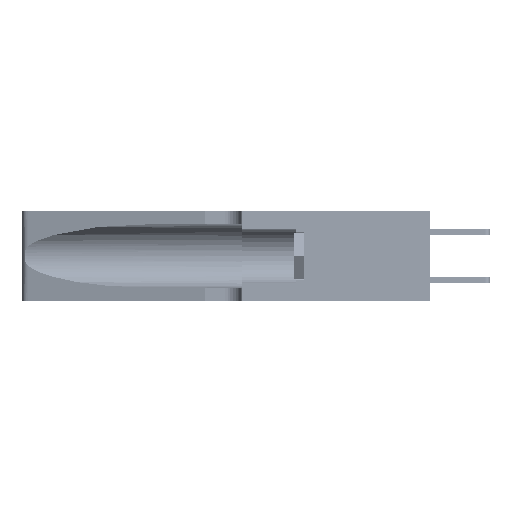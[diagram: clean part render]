
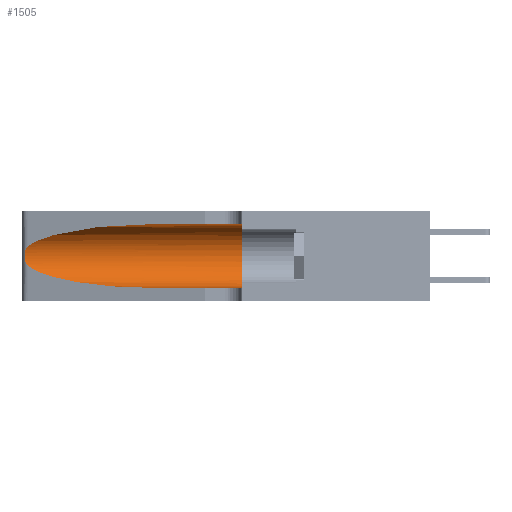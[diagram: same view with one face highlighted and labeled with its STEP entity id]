
A CAD part, left-side view. The second image highlights one B-rep face of the part: STEP entity #1505.
In plain terms, the highlighted cylindrical face has radius 3.308 mm (diameter 6.617 mm), a partial arc.
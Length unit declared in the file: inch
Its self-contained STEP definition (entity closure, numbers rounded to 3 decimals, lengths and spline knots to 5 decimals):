
#581 = DIRECTION ( 'NONE',  ( 0., -1., 0. ) ) ;
#1505 = ADVANCED_FACE ( 'NONE', ( #12681 ), #37578, .F. ) ;
#2303 = B_SPLINE_CURVE_WITH_KNOTS ( 'NONE', 3,
 ( #7524, #19629, #44513, #40163, #36141, #44172, #16311, #28834, #20855, #32813, #32654, #12854, #21021, #8879 ),
 .UNSPECIFIED., .F., .F.,
 ( 4, 2, 2, 2, 2, 2, 4 ),
 ( 0., 0.00027, 0.00053, 0.00107, 0.0016, 0.00187, 0.00214 ),
 .UNSPECIFIED. ) ;
#2967 = VECTOR ( 'NONE', #47442, 39.37008 ) ;
#3426 = ORIENTED_EDGE ( 'NONE', *, *, #32211, .F. ) ;
#5295 = CARTESIAN_POINT ( 'NONE',  ( 0.1305, 0.35, 0.185 ) ) ;
#5371 = ORIENTED_EDGE ( 'NONE', *, *, #38405, .F. ) ;
#5471 = LINE ( 'NONE', #7815, #2967 ) ;
#6158 = LINE ( 'NONE', #24147, #19175 ) ;
#6195 = VERTEX_POINT ( 'NONE', #25731 ) ;
#6636 = CARTESIAN_POINT ( 'NONE',  ( 0.2373, 1.15595, 0.08982 ) ) ;
#7524 = CARTESIAN_POINT ( 'NONE',  ( 0.25487, 1.22718, 0.22369 ) ) ;
#7773 = EDGE_LOOP ( 'NONE', ( #16819, #8786, #22682, #30614, #5371, #3426 ) ) ;
#7815 = CARTESIAN_POINT ( 'NONE',  ( 0.1305, 1.61858, 0.05475 ) ) ;
#8786 = ORIENTED_EDGE ( 'NONE', *, *, #30334, .T. ) ;
#8879 = CARTESIAN_POINT ( 'NONE',  ( 0.25487, 1.22718, 0.14631 ) ) ;
#8909 = DIRECTION ( 'NONE',  ( 0., 0., -1. ) ) ;
#12681 = FACE_OUTER_BOUND ( 'NONE', #7773, .T. ) ;
#12854 = CARTESIAN_POINT ( 'NONE',  ( 0.25639, 1.23186, 0.15144 ) ) ;
#14620 = CARTESIAN_POINT ( 'NONE',  ( 0.1305, 0.72297, 0.05475 ) ) ;
#14790 = CARTESIAN_POINT ( 'NONE',  ( 0.25487, 1.22718, 0.14631 ) ) ;
#15241 = VERTEX_POINT ( 'NONE', #48734 ) ;
#15251 = CARTESIAN_POINT ( 'NONE',  ( 0.25487, 1.22718, 0.22369 ) ) ;
#16311 = CARTESIAN_POINT ( 'NONE',  ( 0.26075, 1.23896, 0.19203 ) ) ;
#16819 = ORIENTED_EDGE ( 'NONE', *, *, #44148, .T. ) ;
#17092 = CARTESIAN_POINT ( 'NONE',  ( 0.1305, 0.35, 0.31525 ) ) ;
#17100 = VERTEX_POINT ( 'NONE', #24023 ) ;
#18113 = VERTEX_POINT ( 'NONE', #41832 ) ;
#19175 = VECTOR ( 'NONE', #581, 39.37008 ) ;
#19629 = CARTESIAN_POINT ( 'NONE',  ( 0.25555, 1.22994, 0.2215 ) ) ;
#20537 = DIRECTION ( 'NONE',  ( 0., -1., 0. ) ) ;
#20797 = VERTEX_POINT ( 'NONE', #17092 ) ;
#20855 = CARTESIAN_POINT ( 'NONE',  ( 0.26017, 1.23833, 0.17102 ) ) ;
#21021 = CARTESIAN_POINT ( 'NONE',  ( 0.25555, 1.22993, 0.14849 ) ) ;
#22682 = ORIENTED_EDGE ( 'NONE', *, *, #30111, .T. ) ;
#24023 = CARTESIAN_POINT ( 'NONE',  ( 0.25487, 1.22718, 0.22369 ) ) ;
#24147 = CARTESIAN_POINT ( 'NONE',  ( 0.1305, 1.61858, 0.31525 ) ) ;
#25731 = CARTESIAN_POINT ( 'NONE',  ( 0.1305, 0.35, 0.05475 ) ) ;
#26421 = CIRCLE ( 'NONE', #28536, 0.13025 ) ;
#27410 = CARTESIAN_POINT ( 'NONE',  ( 0.1305, 0.72297, 0.31525 ) ) ;
#27765 = CARTESIAN_POINT ( 'NONE',  ( 0.1305, 0.72297, 0.05475 ) ) ;
#28536 = AXIS2_PLACEMENT_3D ( 'NONE', #5295, #48743, #37069 ) ;
#28834 = CARTESIAN_POINT ( 'NONE',  ( 0.26075, 1.23896, 0.178 ) ) ;
#30111 = EDGE_CURVE ( 'NONE', #15241, #40724, #45338, .T. ) ;
#30334 = EDGE_CURVE ( 'NONE', #17100, #15241, #2303, .T. ) ;
#30614 = ORIENTED_EDGE ( 'NONE', *, *, #32828, .T. ) ;
#32211 = EDGE_CURVE ( 'NONE', #18113, #20797, #6158, .T. ) ;
#32654 = CARTESIAN_POINT ( 'NONE',  ( 0.25789, 1.23486, 0.15765 ) ) ;
#32813 = CARTESIAN_POINT ( 'NONE',  ( 0.25856, 1.23593, 0.16098 ) ) ;
#32828 = EDGE_CURVE ( 'NONE', #40724, #6195, #5471, .T. ) ;
#34601 = CARTESIAN_POINT ( 'NONE',  ( 0.18966, 0.96281, 0.05475 ) ) ;
#36141 = CARTESIAN_POINT ( 'NONE',  ( 0.25854, 1.2359, 0.20912 ) ) ;
#37069 = DIRECTION ( 'NONE',  ( 0., 0., 1. ) ) ;
#37578 = CYLINDRICAL_SURFACE ( 'NONE', #46438, 0.13025 ) ;
#38405 = EDGE_CURVE ( 'NONE', #20797, #6195, #26421, .T. ) ;
#40163 = CARTESIAN_POINT ( 'NONE',  ( 0.25787, 1.23484, 0.2124 ) ) ;
#40724 = VERTEX_POINT ( 'NONE', #27765 ) ;
#41511 =( BOUNDED_CURVE ( )  B_SPLINE_CURVE ( 3, ( #27410, #50745, #42763, #15251 ),
 .UNSPECIFIED., .F., .F. ) 
 B_SPLINE_CURVE_WITH_KNOTS ( ( 4, 4 ),
 ( 1.5708, 2.84003 ),
 .UNSPECIFIED. ) 
 CURVE ( )  GEOMETRIC_REPRESENTATION_ITEM ( )  RATIONAL_B_SPLINE_CURVE ( ( 1., 0.87, 0.87, 1. ) ) 
 REPRESENTATION_ITEM ( '' )  );
#41832 = CARTESIAN_POINT ( 'NONE',  ( 0.1305, 0.72297, 0.31525 ) ) ;
#42763 = CARTESIAN_POINT ( 'NONE',  ( 0.2373, 1.15595, 0.28018 ) ) ;
#44148 = EDGE_CURVE ( 'NONE', #18113, #17100, #41511, .T. ) ;
#44172 = CARTESIAN_POINT ( 'NONE',  ( 0.26018, 1.23835, 0.19895 ) ) ;
#44513 = CARTESIAN_POINT ( 'NONE',  ( 0.25639, 1.23184, 0.21858 ) ) ;
#45338 =( BOUNDED_CURVE ( )  B_SPLINE_CURVE ( 3, ( #14790, #6636, #34601, #14620 ),
 .UNSPECIFIED., .F., .F. ) 
 B_SPLINE_CURVE_WITH_KNOTS ( ( 4, 4 ),
 ( 3.44316, 4.71239 ),
 .UNSPECIFIED. ) 
 CURVE ( )  GEOMETRIC_REPRESENTATION_ITEM ( )  RATIONAL_B_SPLINE_CURVE ( ( 1., 0.87, 0.87, 1. ) ) 
 REPRESENTATION_ITEM ( '' )  );
#46438 = AXIS2_PLACEMENT_3D ( 'NONE', #48555, #20537, #8909 ) ;
#47442 = DIRECTION ( 'NONE',  ( 0., -1., 0. ) ) ;
#48555 = CARTESIAN_POINT ( 'NONE',  ( 0.1305, 1.61858, 0.185 ) ) ;
#48734 = CARTESIAN_POINT ( 'NONE',  ( 0.25487, 1.22718, 0.14631 ) ) ;
#48743 = DIRECTION ( 'NONE',  ( 0., 1., 0. ) ) ;
#50745 = CARTESIAN_POINT ( 'NONE',  ( 0.18966, 0.96281, 0.31525 ) ) ;
